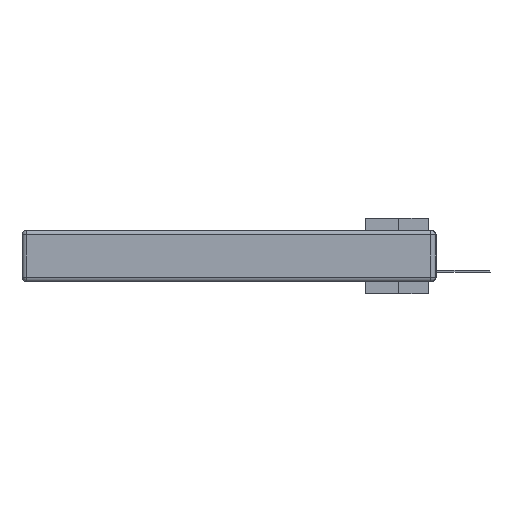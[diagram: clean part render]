
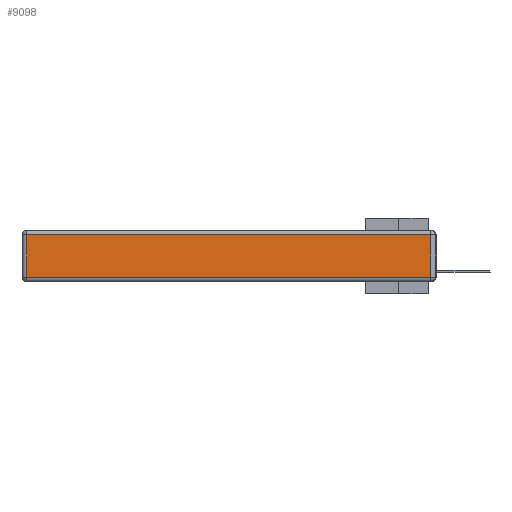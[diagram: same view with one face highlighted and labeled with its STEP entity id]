
A CAD part, left-side view. The second image highlights one B-rep face of the part: STEP entity #9098.
In plain terms, the highlighted planar face has unit normal (-1, 0, 0).
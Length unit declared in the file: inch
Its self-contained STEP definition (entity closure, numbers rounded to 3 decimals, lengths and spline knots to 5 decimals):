
#135 = DIRECTION ( 'NONE',  ( 0., 0., 1. ) ) ;
#938 = VERTEX_POINT ( 'NONE', #36439 ) ;
#1348 = VERTEX_POINT ( 'NONE', #25366 ) ;
#1702 = EDGE_CURVE ( 'NONE', #4643, #938, #30918, .T. ) ;
#2102 = CARTESIAN_POINT ( 'NONE',  ( 0., 2.75, -0.03 ) ) ;
#2141 = EDGE_LOOP ( 'NONE', ( #39148, #11302, #2634, #6583 ) ) ;
#2634 = ORIENTED_EDGE ( 'NONE', *, *, #4203, .T. ) ;
#4203 = EDGE_CURVE ( 'NONE', #26751, #1348, #30394, .T. ) ;
#4643 = VERTEX_POINT ( 'NONE', #18906 ) ;
#6028 = EDGE_CURVE ( 'NONE', #938, #26751, #38893, .T. ) ;
#6414 = LINE ( 'NONE', #25634, #21638 ) ;
#6449 = DIRECTION ( 'NONE',  ( 0., 0., 1. ) ) ;
#6583 = ORIENTED_EDGE ( 'NONE', *, *, #21392, .T. ) ;
#9098 = ADVANCED_FACE ( 'NONE', ( #21769 ), #27902, .T. ) ;
#11302 = ORIENTED_EDGE ( 'NONE', *, *, #6028, .T. ) ;
#11790 = VECTOR ( 'NONE', #33444, 39.37008 ) ;
#13476 = DIRECTION ( 'NONE',  ( 0., 0., -1. ) ) ;
#14152 = VECTOR ( 'NONE', #20558, 39.37008 ) ;
#15134 = CARTESIAN_POINT ( 'NONE',  ( 0., 0.03, -0.343 ) ) ;
#18906 = CARTESIAN_POINT ( 'NONE',  ( 0., 2.72, -0.313 ) ) ;
#18970 = CARTESIAN_POINT ( 'NONE',  ( 0., 0., -0.343 ) ) ;
#20558 = DIRECTION ( 'NONE',  ( 0., 1., 0. ) ) ;
#21392 = EDGE_CURVE ( 'NONE', #1348, #4643, #6414, .T. ) ;
#21638 = VECTOR ( 'NONE', #13476, 39.37008 ) ;
#21769 = FACE_OUTER_BOUND ( 'NONE', #2141, .T. ) ;
#23586 = VECTOR ( 'NONE', #135, 39.37008 ) ;
#24696 = DIRECTION ( 'NONE',  ( -1., 0., 0. ) ) ;
#25366 = CARTESIAN_POINT ( 'NONE',  ( 0., 2.72, -0.03 ) ) ;
#25634 = CARTESIAN_POINT ( 'NONE',  ( 0., 2.72, -0.343 ) ) ;
#26751 = VERTEX_POINT ( 'NONE', #36082 ) ;
#27093 = CARTESIAN_POINT ( 'NONE',  ( 0., 0., -0.313 ) ) ;
#27902 = PLANE ( 'NONE',  #31150 ) ;
#30394 = LINE ( 'NONE', #2102, #14152 ) ;
#30918 = LINE ( 'NONE', #27093, #11790 ) ;
#31150 = AXIS2_PLACEMENT_3D ( 'NONE', #18970, #24696, #6449 ) ;
#33444 = DIRECTION ( 'NONE',  ( 0., -1., 0. ) ) ;
#36082 = CARTESIAN_POINT ( 'NONE',  ( 0., 0.03, -0.03 ) ) ;
#36439 = CARTESIAN_POINT ( 'NONE',  ( 0., 0.03, -0.313 ) ) ;
#38893 = LINE ( 'NONE', #15134, #23586 ) ;
#39148 = ORIENTED_EDGE ( 'NONE', *, *, #1702, .T. ) ;
